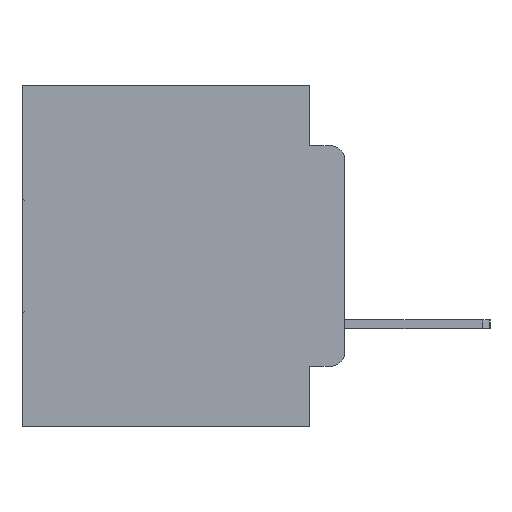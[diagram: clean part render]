
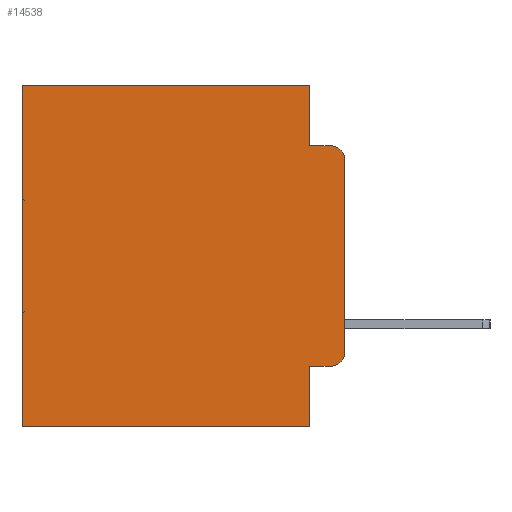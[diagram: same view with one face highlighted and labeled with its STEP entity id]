
A CAD part, left-side view. The second image highlights one B-rep face of the part: STEP entity #14538.
In plain terms, the highlighted planar face has unit normal (-1, 0, 0).
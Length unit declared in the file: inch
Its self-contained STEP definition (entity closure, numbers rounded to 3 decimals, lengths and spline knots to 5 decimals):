
#286 = VERTEX_POINT ( 'NONE', #23354 ) ;
#341 = CARTESIAN_POINT ( 'NONE',  ( 0.298, 0.051, -0.5 ) ) ;
#758 = CARTESIAN_POINT ( 'NONE',  ( 0.298, 0., -0.5 ) ) ;
#833 = ORIENTED_EDGE ( 'NONE', *, *, #22479, .F. ) ;
#1476 = VECTOR ( 'NONE', #15362, 39.37008 ) ;
#1583 = LINE ( 'NONE', #27356, #13777 ) ;
#1928 = DIRECTION ( 'NONE',  ( 0., 0., -1. ) ) ;
#2163 = AXIS2_PLACEMENT_3D ( 'NONE', #26397, #12269, #28777 ) ;
#4015 = ORIENTED_EDGE ( 'NONE', *, *, #10113, .F. ) ;
#4544 = CARTESIAN_POINT ( 'NONE',  ( 0.298, 0.473, -0.5 ) ) ;
#4651 = CARTESIAN_POINT ( 'NONE',  ( 0.298, 0.051, 0. ) ) ;
#4776 = LINE ( 'NONE', #758, #29324 ) ;
#5838 = FACE_OUTER_BOUND ( 'NONE', #14808, .T. ) ;
#5925 = DIRECTION ( 'NONE',  ( 0., 0., -1. ) ) ;
#6219 = EDGE_CURVE ( 'NONE', #17906, #16767, #25945, .T. ) ;
#6423 = VECTOR ( 'NONE', #10357, 39.37008 ) ;
#7218 = LINE ( 'NONE', #7903, #6423 ) ;
#7903 = CARTESIAN_POINT ( 'NONE',  ( 0.298, 0., 0. ) ) ;
#8080 = DIRECTION ( 'NONE',  ( 0., 0., -1. ) ) ;
#8148 = LINE ( 'NONE', #18003, #20120 ) ;
#9765 = CARTESIAN_POINT ( 'NONE',  ( 0.298, 0.473, 0. ) ) ;
#9889 = DIRECTION ( 'NONE',  ( 0., -1., 0. ) ) ;
#9980 = VERTEX_POINT ( 'NONE', #24335 ) ;
#10113 = EDGE_CURVE ( 'NONE', #16916, #20230, #15183, .T. ) ;
#10357 = DIRECTION ( 'NONE',  ( 0., 1., 0. ) ) ;
#10884 = CARTESIAN_POINT ( 'NONE',  ( 0.298, 0.051, 0. ) ) ;
#10974 = EDGE_CURVE ( 'NONE', #16916, #12579, #17082, .T. ) ;
#12269 = DIRECTION ( 'NONE',  ( -1., 0., 0. ) ) ;
#12579 = VERTEX_POINT ( 'NONE', #27739 ) ;
#12735 = EDGE_CURVE ( 'NONE', #17906, #9980, #15424, .T. ) ;
#13088 = DIRECTION ( 'NONE',  ( 0., -1., 0. ) ) ;
#13391 = VECTOR ( 'NONE', #18966, 39.37008 ) ;
#13777 = VECTOR ( 'NONE', #5925, 39.37008 ) ;
#13925 = EDGE_CURVE ( 'NONE', #16767, #29187, #4776, .T. ) ;
#14538 = ADVANCED_FACE ( 'NONE', ( #5838 ), #17629, .F. ) ;
#14653 = ORIENTED_EDGE ( 'NONE', *, *, #29130, .T. ) ;
#14667 = AXIS2_PLACEMENT_3D ( 'NONE', #30529, #16476, #1928 ) ;
#14682 = VECTOR ( 'NONE', #9889, 39.37008 ) ;
#14807 = CARTESIAN_POINT ( 'NONE',  ( 0.298, 0.051, -0.4115 ) ) ;
#14808 = EDGE_LOOP ( 'NONE', ( #4015, #17908, #833, #24521, #23464, #17223, #27448, #27710, #30277, #14653 ) ) ;
#15183 = LINE ( 'NONE', #29445, #1476 ) ;
#15362 = DIRECTION ( 'NONE',  ( 0., 0., -1. ) ) ;
#15424 = LINE ( 'NONE', #19348, #14682 ) ;
#15518 = VERTEX_POINT ( 'NONE', #9765 ) ;
#16476 = DIRECTION ( 'NONE',  ( -1., 0., 0. ) ) ;
#16767 = VERTEX_POINT ( 'NONE', #341 ) ;
#16916 = VERTEX_POINT ( 'NONE', #27178 ) ;
#17082 = CIRCLE ( 'NONE', #2163, 0.02 ) ;
#17223 = ORIENTED_EDGE ( 'NONE', *, *, #19111, .T. ) ;
#17629 = PLANE ( 'NONE',  #17641 ) ;
#17641 = AXIS2_PLACEMENT_3D ( 'NONE', #19992, #22357, #8080 ) ;
#17906 = VERTEX_POINT ( 'NONE', #14807 ) ;
#17908 = ORIENTED_EDGE ( 'NONE', *, *, #10974, .T. ) ;
#18003 = CARTESIAN_POINT ( 'NONE',  ( 0.298, 0.051, -0.0885 ) ) ;
#18966 = DIRECTION ( 'NONE',  ( 0., 0., -1. ) ) ;
#19111 = EDGE_CURVE ( 'NONE', #15518, #29187, #1583, .T. ) ;
#19348 = CARTESIAN_POINT ( 'NONE',  ( 0.298, 0.051, -0.4115 ) ) ;
#19992 = CARTESIAN_POINT ( 'NONE',  ( 0.298, 0., 0. ) ) ;
#20120 = VECTOR ( 'NONE', #13088, 39.37008 ) ;
#20230 = VERTEX_POINT ( 'NONE', #22108 ) ;
#21394 = VECTOR ( 'NONE', #27366, 39.37008 ) ;
#22108 = CARTESIAN_POINT ( 'NONE',  ( 0.298, 0., -0.3915 ) ) ;
#22357 = DIRECTION ( 'NONE',  ( 1., 0., 0. ) ) ;
#22479 = EDGE_CURVE ( 'NONE', #286, #12579, #8148, .T. ) ;
#22491 = DIRECTION ( 'NONE',  ( 0., 1., 0. ) ) ;
#23354 = CARTESIAN_POINT ( 'NONE',  ( 0.298, 0.051, -0.0885 ) ) ;
#23464 = ORIENTED_EDGE ( 'NONE', *, *, #30049, .T. ) ;
#24335 = CARTESIAN_POINT ( 'NONE',  ( 0.298, 0.02, -0.4115 ) ) ;
#24521 = ORIENTED_EDGE ( 'NONE', *, *, #30331, .F. ) ;
#25485 = CIRCLE ( 'NONE', #14667, 0.02 ) ;
#25945 = LINE ( 'NONE', #28286, #13391 ) ;
#26397 = CARTESIAN_POINT ( 'NONE',  ( 0.298, 0.02, -0.1085 ) ) ;
#26743 = VERTEX_POINT ( 'NONE', #4651 ) ;
#27178 = CARTESIAN_POINT ( 'NONE',  ( 0.298, 0., -0.1085 ) ) ;
#27356 = CARTESIAN_POINT ( 'NONE',  ( 0.298, 0.473, 0. ) ) ;
#27366 = DIRECTION ( 'NONE',  ( 0., 0., -1. ) ) ;
#27448 = ORIENTED_EDGE ( 'NONE', *, *, #13925, .F. ) ;
#27609 = LINE ( 'NONE', #10884, #21394 ) ;
#27710 = ORIENTED_EDGE ( 'NONE', *, *, #6219, .F. ) ;
#27739 = CARTESIAN_POINT ( 'NONE',  ( 0.298, 0.02, -0.0885 ) ) ;
#28286 = CARTESIAN_POINT ( 'NONE',  ( 0.298, 0.051, 0. ) ) ;
#28777 = DIRECTION ( 'NONE',  ( 0., 0., -1. ) ) ;
#29130 = EDGE_CURVE ( 'NONE', #9980, #20230, #25485, .T. ) ;
#29187 = VERTEX_POINT ( 'NONE', #4544 ) ;
#29324 = VECTOR ( 'NONE', #22491, 39.37008 ) ;
#29445 = CARTESIAN_POINT ( 'NONE',  ( 0.298, 0., 0. ) ) ;
#30049 = EDGE_CURVE ( 'NONE', #26743, #15518, #7218, .T. ) ;
#30277 = ORIENTED_EDGE ( 'NONE', *, *, #12735, .T. ) ;
#30331 = EDGE_CURVE ( 'NONE', #26743, #286, #27609, .T. ) ;
#30529 = CARTESIAN_POINT ( 'NONE',  ( 0.298, 0.02, -0.3915 ) ) ;
